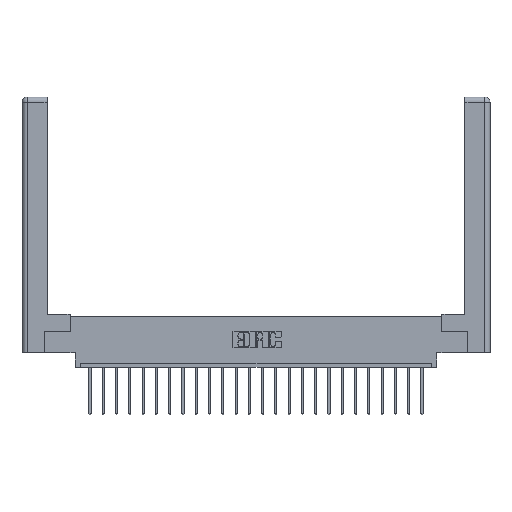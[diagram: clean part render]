
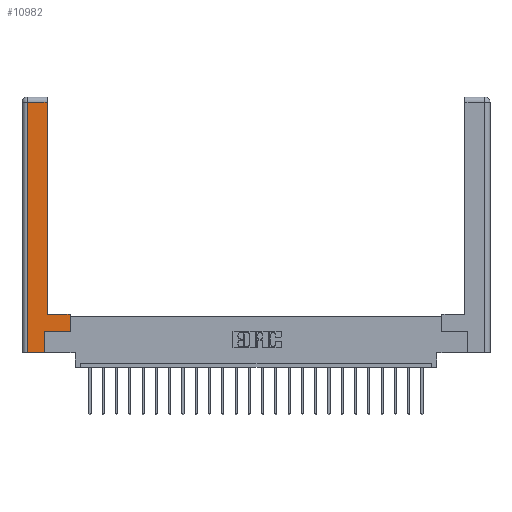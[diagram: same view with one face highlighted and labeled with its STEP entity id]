
A CAD part, top view. The second image highlights one B-rep face of the part: STEP entity #10982.
In plain terms, the highlighted planar face has unit normal (0, 0, 1).
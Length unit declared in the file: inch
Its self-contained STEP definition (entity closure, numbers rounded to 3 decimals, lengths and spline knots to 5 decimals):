
#572 = VECTOR ( 'NONE', #9710, 39.37008 ) ;
#1863 = EDGE_CURVE ( 'NONE', #2553, #11788, #13502, .T. ) ;
#2290 = CARTESIAN_POINT ( 'NONE',  ( 0.265, 0., 0. ) ) ;
#2553 = VERTEX_POINT ( 'NONE', #3756 ) ;
#3457 = ORIENTED_EDGE ( 'NONE', *, *, #15947, .T. ) ;
#3669 = EDGE_CURVE ( 'NONE', #18009, #12913, #12510, .T. ) ;
#3716 = FACE_OUTER_BOUND ( 'NONE', #21433, .T. ) ;
#3756 = CARTESIAN_POINT ( 'NONE',  ( 0.565, 0.45, 0. ) ) ;
#3784 = VERTEX_POINT ( 'NONE', #15602 ) ;
#4124 = CARTESIAN_POINT ( 'NONE',  ( 0.0615, 0., 0. ) ) ;
#4172 = EDGE_CURVE ( 'NONE', #5588, #8525, #13660, .T. ) ;
#4364 = LINE ( 'NONE', #19344, #22454 ) ;
#4670 = VECTOR ( 'NONE', #8611, 39.37008 ) ;
#5239 = DIRECTION ( 'NONE',  ( 1., 0., 0. ) ) ;
#5588 = VERTEX_POINT ( 'NONE', #2290 ) ;
#5683 = CARTESIAN_POINT ( 'NONE',  ( 0.565, 0.245, 0. ) ) ;
#6013 = CARTESIAN_POINT ( 'NONE',  ( 0.0615, 2.94, 0. ) ) ;
#6199 = PLANE ( 'NONE',  #6697 ) ;
#6344 = CARTESIAN_POINT ( 'NONE',  ( 0.0615, 0., 0. ) ) ;
#6697 = AXIS2_PLACEMENT_3D ( 'NONE', #19033, #18959, #11815 ) ;
#7219 = ORIENTED_EDGE ( 'NONE', *, *, #16626, .T. ) ;
#7222 = CARTESIAN_POINT ( 'NONE',  ( 0.295, 0.45, 0. ) ) ;
#8013 = DIRECTION ( 'NONE',  ( 0., 1., 0. ) ) ;
#8371 = DIRECTION ( 'NONE',  ( -1., 0., 0. ) ) ;
#8525 = VERTEX_POINT ( 'NONE', #20522 ) ;
#8543 = CARTESIAN_POINT ( 'NONE',  ( 0.295, 3., 0. ) ) ;
#8611 = DIRECTION ( 'NONE',  ( 0., 1., 0. ) ) ;
#9187 = DIRECTION ( 'NONE',  ( 0., 1., 0. ) ) ;
#9710 = DIRECTION ( 'NONE',  ( 0., -1., 0. ) ) ;
#9893 = EDGE_CURVE ( 'NONE', #23449, #2553, #4364, .T. ) ;
#10179 = LINE ( 'NONE', #19878, #11041 ) ;
#10874 = VECTOR ( 'NONE', #18408, 39.37008 ) ;
#10908 = VECTOR ( 'NONE', #14895, 39.37008 ) ;
#10982 = ADVANCED_FACE ( 'NONE', ( #3716 ), #6199, .F. ) ;
#11041 = VECTOR ( 'NONE', #5239, 39.37008 ) ;
#11096 = CARTESIAN_POINT ( 'NONE',  ( 0.565, 0.245, 0. ) ) ;
#11135 = CARTESIAN_POINT ( 'NONE',  ( 0.265, 0.245, 0. ) ) ;
#11651 = LINE ( 'NONE', #12271, #19768 ) ;
#11788 = VERTEX_POINT ( 'NONE', #22951 ) ;
#11815 = DIRECTION ( 'NONE',  ( -1., 0., 0. ) ) ;
#12271 = CARTESIAN_POINT ( 'NONE',  ( 0.0615, 2.94, 0. ) ) ;
#12488 = VECTOR ( 'NONE', #9187, 39.37008 ) ;
#12510 = LINE ( 'NONE', #4124, #572 ) ;
#12522 = ORIENTED_EDGE ( 'NONE', *, *, #3669, .T. ) ;
#12913 = VERTEX_POINT ( 'NONE', #6344 ) ;
#13379 = ORIENTED_EDGE ( 'NONE', *, *, #1863, .T. ) ;
#13502 = LINE ( 'NONE', #7222, #10874 ) ;
#13660 = LINE ( 'NONE', #11135, #12488 ) ;
#14895 = DIRECTION ( 'NONE',  ( 1., 0., 0. ) ) ;
#15602 = CARTESIAN_POINT ( 'NONE',  ( 0.295, 2.94, 0. ) ) ;
#15851 = ORIENTED_EDGE ( 'NONE', *, *, #20465, .T. ) ;
#15947 = EDGE_CURVE ( 'NONE', #3784, #18009, #11651, .T. ) ;
#16626 = EDGE_CURVE ( 'NONE', #12913, #5588, #10179, .T. ) ;
#16886 = ORIENTED_EDGE ( 'NONE', *, *, #19221, .T. ) ;
#18009 = VERTEX_POINT ( 'NONE', #6013 ) ;
#18408 = DIRECTION ( 'NONE',  ( -1., 0., 0. ) ) ;
#18959 = DIRECTION ( 'NONE',  ( 0., 0., -1. ) ) ;
#19033 = CARTESIAN_POINT ( 'NONE',  ( 0., 0., 0. ) ) ;
#19221 = EDGE_CURVE ( 'NONE', #8525, #23449, #20830, .T. ) ;
#19344 = CARTESIAN_POINT ( 'NONE',  ( 0.565, 0.45, 0. ) ) ;
#19768 = VECTOR ( 'NONE', #8371, 39.37008 ) ;
#19878 = CARTESIAN_POINT ( 'NONE',  ( 0.265, 0., 0. ) ) ;
#20465 = EDGE_CURVE ( 'NONE', #11788, #3784, #23355, .T. ) ;
#20522 = CARTESIAN_POINT ( 'NONE',  ( 0.265, 0.245, 0. ) ) ;
#20830 = LINE ( 'NONE', #11096, #10908 ) ;
#20895 = ORIENTED_EDGE ( 'NONE', *, *, #4172, .T. ) ;
#21433 = EDGE_LOOP ( 'NONE', ( #15851, #3457, #12522, #7219, #20895, #16886, #22722, #13379 ) ) ;
#22454 = VECTOR ( 'NONE', #8013, 39.37008 ) ;
#22722 = ORIENTED_EDGE ( 'NONE', *, *, #9893, .T. ) ;
#22951 = CARTESIAN_POINT ( 'NONE',  ( 0.295, 0.45, 0. ) ) ;
#23355 = LINE ( 'NONE', #8543, #4670 ) ;
#23449 = VERTEX_POINT ( 'NONE', #5683 ) ;
